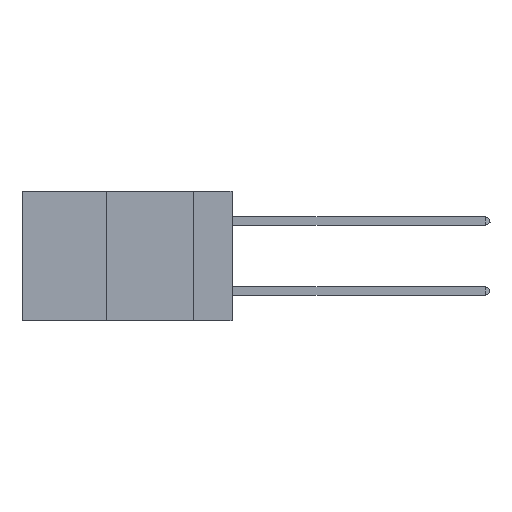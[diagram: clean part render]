
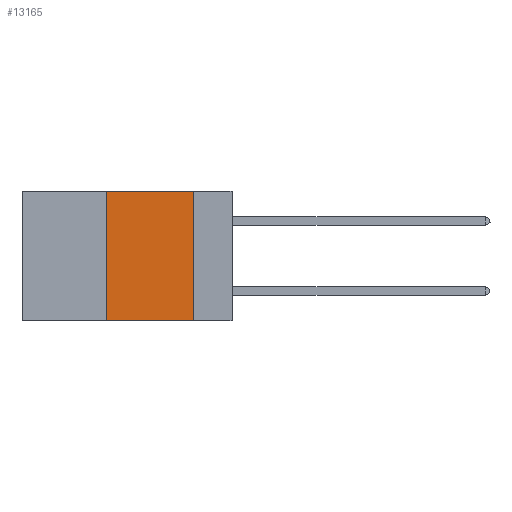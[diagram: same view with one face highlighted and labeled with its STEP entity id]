
A CAD part, left-side view. The second image highlights one B-rep face of the part: STEP entity #13165.
In plain terms, the highlighted planar face has unit normal (-1, 0, 0).
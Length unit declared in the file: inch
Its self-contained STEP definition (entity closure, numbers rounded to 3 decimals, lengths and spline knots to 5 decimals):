
#846 = EDGE_CURVE ( 'NONE', #10689, #5120, #10996, .T. ) ;
#2071 = ORIENTED_EDGE ( 'NONE', *, *, #846, .T. ) ;
#2076 = LINE ( 'NONE', #5676, #21842 ) ;
#4285 = VECTOR ( 'NONE', #16411, 39.37008 ) ;
#4781 = LINE ( 'NONE', #15606, #17604 ) ;
#5109 = DIRECTION ( 'NONE',  ( 0., 0., -1. ) ) ;
#5120 = VERTEX_POINT ( 'NONE', #12099 ) ;
#5620 = VERTEX_POINT ( 'NONE', #21291 ) ;
#5676 = CARTESIAN_POINT ( 'NONE',  ( 0., 0.6, 0. ) ) ;
#7110 = CARTESIAN_POINT ( 'NONE',  ( 0., 0.36, 0. ) ) ;
#7262 = EDGE_LOOP ( 'NONE', ( #17750, #16965, #9586, #2071 ) ) ;
#7526 = VERTEX_POINT ( 'NONE', #17994 ) ;
#7899 = EDGE_CURVE ( 'NONE', #7526, #5620, #2076, .T. ) ;
#9586 = ORIENTED_EDGE ( 'NONE', *, *, #15997, .F. ) ;
#9647 = AXIS2_PLACEMENT_3D ( 'NONE', #17859, #15677, #5109 ) ;
#9818 = EDGE_CURVE ( 'NONE', #5620, #5120, #4781, .T. ) ;
#10689 = VERTEX_POINT ( 'NONE', #23039 ) ;
#10996 = LINE ( 'NONE', #18342, #4285 ) ;
#11762 = DIRECTION ( 'NONE',  ( 0., 0., -1. ) ) ;
#12099 = CARTESIAN_POINT ( 'NONE',  ( 0., 0.11, -0.37 ) ) ;
#13165 = ADVANCED_FACE ( 'NONE', ( #15810 ), #17745, .F. ) ;
#15606 = CARTESIAN_POINT ( 'NONE',  ( 0., 0.11, 0. ) ) ;
#15677 = DIRECTION ( 'NONE',  ( 1., 0., 0. ) ) ;
#15810 = FACE_OUTER_BOUND ( 'NONE', #7262, .T. ) ;
#15997 = EDGE_CURVE ( 'NONE', #10689, #7526, #23505, .T. ) ;
#16411 = DIRECTION ( 'NONE',  ( 0., -1., 0. ) ) ;
#16965 = ORIENTED_EDGE ( 'NONE', *, *, #7899, .F. ) ;
#17604 = VECTOR ( 'NONE', #11762, 39.37008 ) ;
#17745 = PLANE ( 'NONE',  #9647 ) ;
#17750 = ORIENTED_EDGE ( 'NONE', *, *, #9818, .F. ) ;
#17859 = CARTESIAN_POINT ( 'NONE',  ( 0., 0.6, 0. ) ) ;
#17994 = CARTESIAN_POINT ( 'NONE',  ( 0., 0.36, 0. ) ) ;
#18192 = VECTOR ( 'NONE', #18307, 39.37008 ) ;
#18307 = DIRECTION ( 'NONE',  ( 0., 0., 1. ) ) ;
#18342 = CARTESIAN_POINT ( 'NONE',  ( 0., 0.6, -0.37 ) ) ;
#21291 = CARTESIAN_POINT ( 'NONE',  ( 0., 0.11, 0. ) ) ;
#21842 = VECTOR ( 'NONE', #22423, 39.37008 ) ;
#22423 = DIRECTION ( 'NONE',  ( 0., -1., 0. ) ) ;
#23039 = CARTESIAN_POINT ( 'NONE',  ( 0., 0.36, -0.37 ) ) ;
#23505 = LINE ( 'NONE', #7110, #18192 ) ;
